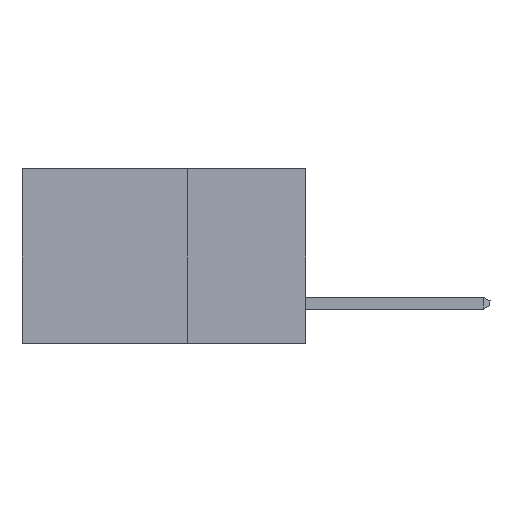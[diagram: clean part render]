
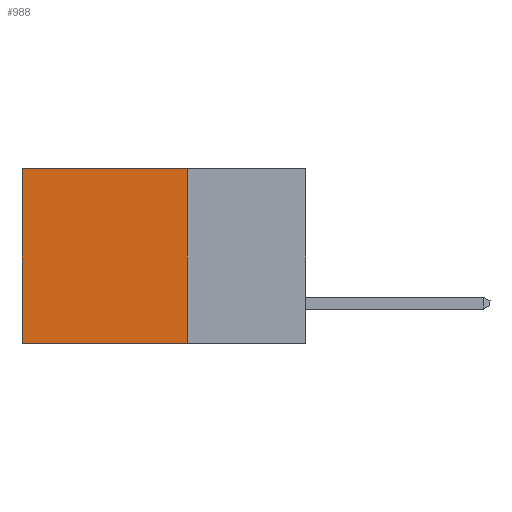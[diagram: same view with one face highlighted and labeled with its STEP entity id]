
A CAD part, left-side view. The second image highlights one B-rep face of the part: STEP entity #988.
In plain terms, the highlighted planar face has unit normal (-1, 0, 0).
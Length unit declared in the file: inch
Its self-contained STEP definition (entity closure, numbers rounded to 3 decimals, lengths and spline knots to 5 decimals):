
#366 = CARTESIAN_POINT ( 'NONE',  ( 0.2615, 0.25, 0. ) ) ;
#713 = EDGE_LOOP ( 'NONE', ( #15315, #11947, #6324, #8850 ) ) ;
#988 = ADVANCED_FACE ( 'NONE', ( #3863 ), #15259, .F. ) ;
#1268 = VERTEX_POINT ( 'NONE', #7747 ) ;
#2407 = CARTESIAN_POINT ( 'NONE',  ( 0.2615, 0.6, -0.37 ) ) ;
#2870 = VERTEX_POINT ( 'NONE', #3584 ) ;
#3210 = VECTOR ( 'NONE', #6000, 39.37008 ) ;
#3275 = CARTESIAN_POINT ( 'NONE',  ( 0.2615, 0.25, 0. ) ) ;
#3584 = CARTESIAN_POINT ( 'NONE',  ( 0.2615, 0.6, -0.37 ) ) ;
#3863 = FACE_OUTER_BOUND ( 'NONE', #713, .T. ) ;
#4240 = DIRECTION ( 'NONE',  ( 0., 1., 0. ) ) ;
#4614 = CARTESIAN_POINT ( 'NONE',  ( 0.2615, 0.25, -0.37 ) ) ;
#5208 = CARTESIAN_POINT ( 'NONE',  ( 0.2615, 0.25, -0.37 ) ) ;
#6000 = DIRECTION ( 'NONE',  ( 0., 1., 0. ) ) ;
#6169 = DIRECTION ( 'NONE',  ( 0., 0., -1. ) ) ;
#6202 = DIRECTION ( 'NONE',  ( 0., 0., -1. ) ) ;
#6324 = ORIENTED_EDGE ( 'NONE', *, *, #16214, .F. ) ;
#7747 = CARTESIAN_POINT ( 'NONE',  ( 0.2615, 0.6, 0. ) ) ;
#8090 = DIRECTION ( 'NONE',  ( 0., 0., -1. ) ) ;
#8264 = CARTESIAN_POINT ( 'NONE',  ( 0.2615, 0.25, -0.37 ) ) ;
#8850 = ORIENTED_EDGE ( 'NONE', *, *, #9332, .T. ) ;
#9332 = EDGE_CURVE ( 'NONE', #9645, #1268, #11777, .T. ) ;
#9645 = VERTEX_POINT ( 'NONE', #3275 ) ;
#10096 = DIRECTION ( 'NONE',  ( 1., 0., 0. ) ) ;
#10603 = EDGE_CURVE ( 'NONE', #15471, #2870, #16932, .T. ) ;
#11777 = LINE ( 'NONE', #366, #3210 ) ;
#11947 = ORIENTED_EDGE ( 'NONE', *, *, #10603, .F. ) ;
#12521 = LINE ( 'NONE', #2407, #17085 ) ;
#14422 = VECTOR ( 'NONE', #6202, 39.37008 ) ;
#14619 = LINE ( 'NONE', #16098, #14422 ) ;
#15259 = PLANE ( 'NONE',  #15828 ) ;
#15315 = ORIENTED_EDGE ( 'NONE', *, *, #17695, .T. ) ;
#15471 = VERTEX_POINT ( 'NONE', #5208 ) ;
#15828 = AXIS2_PLACEMENT_3D ( 'NONE', #8264, #10096, #6169 ) ;
#16098 = CARTESIAN_POINT ( 'NONE',  ( 0.2615, 0.25, -0.37 ) ) ;
#16214 = EDGE_CURVE ( 'NONE', #9645, #15471, #14619, .T. ) ;
#16932 = LINE ( 'NONE', #4614, #17303 ) ;
#17085 = VECTOR ( 'NONE', #8090, 39.37008 ) ;
#17303 = VECTOR ( 'NONE', #4240, 39.37008 ) ;
#17695 = EDGE_CURVE ( 'NONE', #1268, #2870, #12521, .T. ) ;
